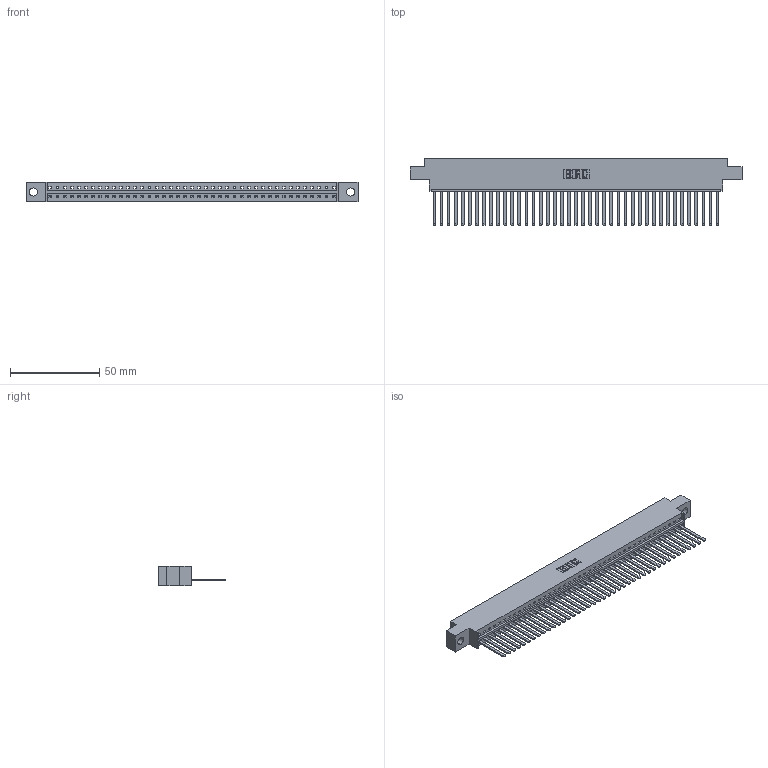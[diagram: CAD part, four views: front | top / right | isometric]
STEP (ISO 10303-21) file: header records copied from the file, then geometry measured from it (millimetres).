
FILE_DESCRIPTION (( 'STEP AP203' ), '1' );
FILE_NAME ('336-041-541-609.STEP', '2020-08-07T23:30:37', ( '' ), ( '' ), 'SwSTEP 2.0', 'SolidWorks 2020', '' );
FILE_SCHEMA (( 'CONFIG_CONTROL_DESIGN' ));
Length unit declared in the file: inch
Products named in the file (3): 336-041-541-609; 336 Part_Offset - .178 Dia - TH; 336-290-001_336-290-541
Assembly tree (42 placements, depth 2):
  336-041-541-609
    336 Part_Offset - .178 Dia - TH
    336-290-001_336-290-541  x41
Bounding box: 185.85 x 37.34 x 11.1 mm (x, y, z)
Volume: 26907.6 mm3; surface area: 29224.8 mm2
Topology: 42 solids, 42 shells, 2168 faces, 6637 edges, 4396 vertices
Faces by surface type: plane 1468, cylinder 700
Entity records: 30460 total; most frequent: CARTESIAN_POINT 5396, ORIENTED_EDGE 5274, DIRECTION 4447, EDGE_CURVE 2637, VECTOR 2505, LINE 2505, VERTEX_POINT 1756, AXIS2_PLACEMENT_3D 971
